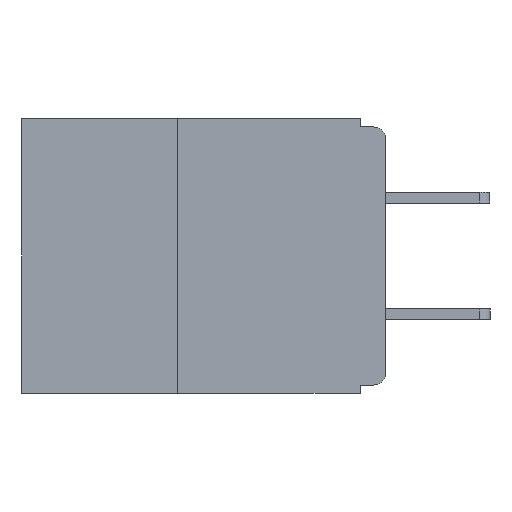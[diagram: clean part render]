
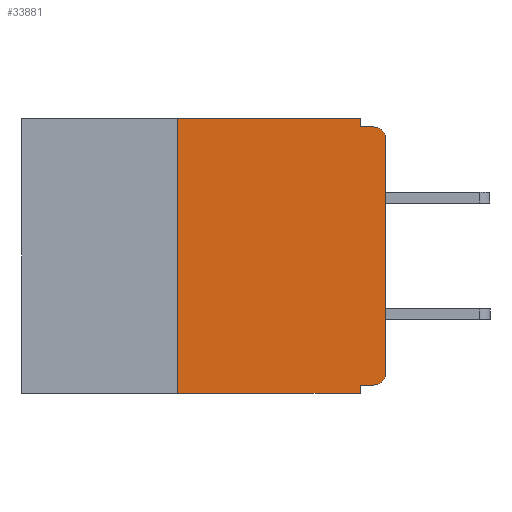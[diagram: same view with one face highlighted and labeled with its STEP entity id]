
A CAD part, left-side view. The second image highlights one B-rep face of the part: STEP entity #33881.
In plain terms, the highlighted planar face has unit normal (-1, 0, 0).
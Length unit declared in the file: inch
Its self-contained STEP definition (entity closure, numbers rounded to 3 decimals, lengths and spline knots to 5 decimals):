
#155 = DIRECTION ( 'NONE',  ( 0., -1., 0. ) ) ;
#332 = CARTESIAN_POINT ( 'NONE',  ( 0., 0., -0.305 ) ) ;
#413 = CARTESIAN_POINT ( 'NONE',  ( 0., 0.437, 0. ) ) ;
#428 = CARTESIAN_POINT ( 'NONE',  ( 0., 0.031, 0. ) ) ;
#790 = DIRECTION ( 'NONE',  ( 0., 0., 1. ) ) ;
#1462 = VERTEX_POINT ( 'NONE', #332 ) ;
#1470 = EDGE_CURVE ( 'NONE', #27589, #20501, #14905, .T. ) ;
#2671 = CARTESIAN_POINT ( 'NONE',  ( 0., 0.015, -0.32 ) ) ;
#3061 = DIRECTION ( 'NONE',  ( 0., 0., -1. ) ) ;
#3448 = LINE ( 'NONE', #428, #31222 ) ;
#3625 = VERTEX_POINT ( 'NONE', #18967 ) ;
#4164 = VECTOR ( 'NONE', #31818, 39.37008 ) ;
#4487 = DIRECTION ( 'NONE',  ( 0., 0., 1. ) ) ;
#5741 = CARTESIAN_POINT ( 'NONE',  ( 0., 0., -0.32 ) ) ;
#7512 = DIRECTION ( 'NONE',  ( -1., 0., 0. ) ) ;
#8011 = CARTESIAN_POINT ( 'NONE',  ( 0., 0., -0.01 ) ) ;
#9050 = EDGE_CURVE ( 'NONE', #18442, #30027, #29489, .T. ) ;
#9354 = AXIS2_PLACEMENT_3D ( 'NONE', #29859, #13999, #32432 ) ;
#9389 = CARTESIAN_POINT ( 'NONE',  ( 0., 0.25, -0.33 ) ) ;
#10575 = CARTESIAN_POINT ( 'NONE',  ( 0., 0.437, -0.33 ) ) ;
#10610 = VECTOR ( 'NONE', #790, 39.37008 ) ;
#11812 = CARTESIAN_POINT ( 'NONE',  ( 0., 0.437, 0. ) ) ;
#13039 = VECTOR ( 'NONE', #16274, 39.37008 ) ;
#13565 = EDGE_CURVE ( 'NONE', #20501, #3625, #3448, .T. ) ;
#13711 = CARTESIAN_POINT ( 'NONE',  ( 0., 0.031, -0.33 ) ) ;
#13999 = DIRECTION ( 'NONE',  ( -1., 0., 0. ) ) ;
#14544 = DIRECTION ( 'NONE',  ( 1., 0., 0. ) ) ;
#14905 = LINE ( 'NONE', #413, #28211 ) ;
#15178 = AXIS2_PLACEMENT_3D ( 'NONE', #23757, #7512, #26357 ) ;
#15301 = CIRCLE ( 'NONE', #15178, 0.015 ) ;
#15593 = EDGE_CURVE ( 'NONE', #1462, #17202, #31794, .T. ) ;
#16046 = CARTESIAN_POINT ( 'NONE',  ( 0., 0.031, 0. ) ) ;
#16274 = DIRECTION ( 'NONE',  ( 0., -1., 0. ) ) ;
#16371 = CIRCLE ( 'NONE', #9354, 0.015 ) ;
#16751 = ORIENTED_EDGE ( 'NONE', *, *, #15593, .T. ) ;
#16792 = VERTEX_POINT ( 'NONE', #9389 ) ;
#16844 = CARTESIAN_POINT ( 'NONE',  ( 0., 0.031, -0.32 ) ) ;
#17202 = VERTEX_POINT ( 'NONE', #22201 ) ;
#17729 = EDGE_CURVE ( 'NONE', #3625, #23208, #28045, .T. ) ;
#18369 = ORIENTED_EDGE ( 'NONE', *, *, #19628, .T. ) ;
#18442 = VERTEX_POINT ( 'NONE', #2671 ) ;
#18967 = CARTESIAN_POINT ( 'NONE',  ( 0., 0.031, -0.01 ) ) ;
#19628 = EDGE_CURVE ( 'NONE', #17202, #23208, #16371, .T. ) ;
#20501 = VERTEX_POINT ( 'NONE', #16046 ) ;
#20941 = CARTESIAN_POINT ( 'NONE',  ( 0., 0.25, -0.33 ) ) ;
#21561 = EDGE_CURVE ( 'NONE', #16792, #27589, #34306, .T. ) ;
#22085 = ORIENTED_EDGE ( 'NONE', *, *, #17729, .F. ) ;
#22201 = CARTESIAN_POINT ( 'NONE',  ( 0., 0., -0.025 ) ) ;
#22259 = CARTESIAN_POINT ( 'NONE',  ( 0., 0.031, -0.33 ) ) ;
#22863 = ORIENTED_EDGE ( 'NONE', *, *, #13565, .F. ) ;
#22883 = EDGE_CURVE ( 'NONE', #18442, #1462, #15301, .T. ) ;
#22950 = CARTESIAN_POINT ( 'NONE',  ( 0., 0.25, 0. ) ) ;
#23107 = VERTEX_POINT ( 'NONE', #13711 ) ;
#23208 = VERTEX_POINT ( 'NONE', #32490 ) ;
#23431 = VECTOR ( 'NONE', #32484, 39.37008 ) ;
#23757 = CARTESIAN_POINT ( 'NONE',  ( 0., 0.015, -0.305 ) ) ;
#24468 = ORIENTED_EDGE ( 'NONE', *, *, #1470, .F. ) ;
#25033 = DIRECTION ( 'NONE',  ( 0., 0., -1. ) ) ;
#25055 = ORIENTED_EDGE ( 'NONE', *, *, #21561, .F. ) ;
#25514 = ORIENTED_EDGE ( 'NONE', *, *, #29219, .T. ) ;
#26000 = ORIENTED_EDGE ( 'NONE', *, *, #33774, .F. ) ;
#26357 = DIRECTION ( 'NONE',  ( 0., 0., -1. ) ) ;
#26362 = LINE ( 'NONE', #22259, #32378 ) ;
#27325 = AXIS2_PLACEMENT_3D ( 'NONE', #11812, #14544, #32957 ) ;
#27589 = VERTEX_POINT ( 'NONE', #22950 ) ;
#27819 = PLANE ( 'NONE',  #27325 ) ;
#28045 = LINE ( 'NONE', #8011, #13039 ) ;
#28211 = VECTOR ( 'NONE', #155, 39.37008 ) ;
#29219 = EDGE_CURVE ( 'NONE', #16792, #23107, #32665, .T. ) ;
#29489 = LINE ( 'NONE', #5741, #23431 ) ;
#29622 = ORIENTED_EDGE ( 'NONE', *, *, #9050, .F. ) ;
#29859 = CARTESIAN_POINT ( 'NONE',  ( 0., 0.015, -0.025 ) ) ;
#29963 = FACE_OUTER_BOUND ( 'NONE', #31945, .T. ) ;
#30027 = VERTEX_POINT ( 'NONE', #16844 ) ;
#30436 = CARTESIAN_POINT ( 'NONE',  ( 0., 0., 0. ) ) ;
#31222 = VECTOR ( 'NONE', #25033, 39.37008 ) ;
#31547 = ORIENTED_EDGE ( 'NONE', *, *, #22883, .T. ) ;
#31794 = LINE ( 'NONE', #30436, #10610 ) ;
#31818 = DIRECTION ( 'NONE',  ( 0., -1., 0. ) ) ;
#31945 = EDGE_LOOP ( 'NONE', ( #16751, #18369, #22085, #22863, #24468, #25055, #25514, #26000, #29622, #31547 ) ) ;
#32378 = VECTOR ( 'NONE', #3061, 39.37008 ) ;
#32432 = DIRECTION ( 'NONE',  ( 0., 0., -1. ) ) ;
#32484 = DIRECTION ( 'NONE',  ( 0., 1., 0. ) ) ;
#32490 = CARTESIAN_POINT ( 'NONE',  ( 0., 0.015, -0.01 ) ) ;
#32665 = LINE ( 'NONE', #10575, #4164 ) ;
#32957 = DIRECTION ( 'NONE',  ( 0., 0., -1. ) ) ;
#33774 = EDGE_CURVE ( 'NONE', #30027, #23107, #26362, .T. ) ;
#33881 = ADVANCED_FACE ( 'NONE', ( #29963 ), #27819, .F. ) ;
#34306 = LINE ( 'NONE', #20941, #34668 ) ;
#34668 = VECTOR ( 'NONE', #4487, 39.37008 ) ;
